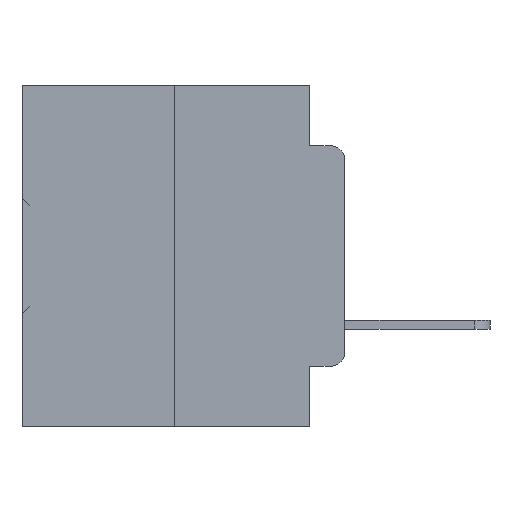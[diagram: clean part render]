
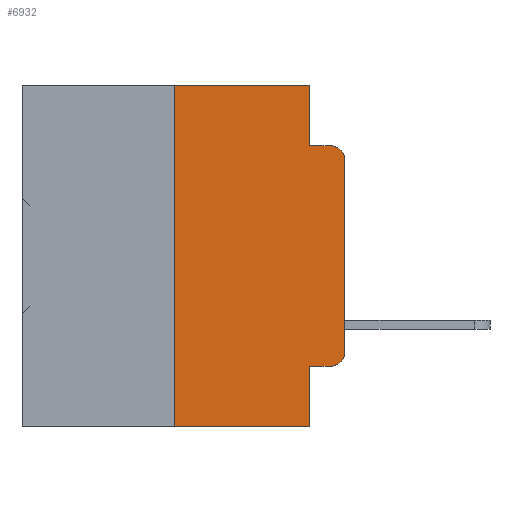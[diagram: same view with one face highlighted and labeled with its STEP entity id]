
A CAD part, left-side view. The second image highlights one B-rep face of the part: STEP entity #6932.
In plain terms, the highlighted planar face has unit normal (-1, 0, 0).
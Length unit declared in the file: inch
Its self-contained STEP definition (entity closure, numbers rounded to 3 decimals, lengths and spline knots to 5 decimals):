
#1112 = ORIENTED_EDGE ( 'NONE', *, *, #26178, .T. ) ;
#2345 = CARTESIAN_POINT ( 'NONE',  ( 0., 0.051, -0.0885 ) ) ;
#2995 = EDGE_CURVE ( 'NONE', #19259, #22812, #21436, .T. ) ;
#3090 = DIRECTION ( 'NONE',  ( 0., 0., -1. ) ) ;
#3223 = ORIENTED_EDGE ( 'NONE', *, *, #34091, .F. ) ;
#3298 = VECTOR ( 'NONE', #9913, 39.37008 ) ;
#3978 = CARTESIAN_POINT ( 'NONE',  ( 0., 0.051, 0. ) ) ;
#4109 = VECTOR ( 'NONE', #13812, 39.37008 ) ;
#4898 = CARTESIAN_POINT ( 'NONE',  ( 0., 0.25, 0. ) ) ;
#5034 = EDGE_CURVE ( 'NONE', #5572, #13903, #10807, .T. ) ;
#5572 = VERTEX_POINT ( 'NONE', #36904 ) ;
#5828 = CARTESIAN_POINT ( 'NONE',  ( 0., 0.25, -0.5 ) ) ;
#6393 = CARTESIAN_POINT ( 'NONE',  ( 0., 0.051, -0.4115 ) ) ;
#6932 = ADVANCED_FACE ( 'NONE', ( #32991 ), #20229, .F. ) ;
#7000 = DIRECTION ( 'NONE',  ( 0., 0., -1. ) ) ;
#7051 = EDGE_CURVE ( 'NONE', #13903, #15037, #23560, .T. ) ;
#7259 = CARTESIAN_POINT ( 'NONE',  ( 0., 0.051, -0.5 ) ) ;
#7495 = AXIS2_PLACEMENT_3D ( 'NONE', #26180, #7966, #29075 ) ;
#7966 = DIRECTION ( 'NONE',  ( 1., 0., 0. ) ) ;
#8162 = CARTESIAN_POINT ( 'NONE',  ( 0., 0.051, -0.4115 ) ) ;
#8817 = ORIENTED_EDGE ( 'NONE', *, *, #2995, .F. ) ;
#9519 = DIRECTION ( 'NONE',  ( 0., -1., 0. ) ) ;
#9913 = DIRECTION ( 'NONE',  ( 0., -1., 0. ) ) ;
#9925 = CARTESIAN_POINT ( 'NONE',  ( 0., 0., -0.3915 ) ) ;
#10504 = DIRECTION ( 'NONE',  ( 0., 0., -1. ) ) ;
#10753 = CARTESIAN_POINT ( 'NONE',  ( 0., 0.473, 0. ) ) ;
#10807 = LINE ( 'NONE', #3978, #38237 ) ;
#11054 = ORIENTED_EDGE ( 'NONE', *, *, #7051, .F. ) ;
#11085 = CARTESIAN_POINT ( 'NONE',  ( 0., 0.02, -0.0885 ) ) ;
#11275 = EDGE_CURVE ( 'NONE', #12310, #15037, #15644, .T. ) ;
#11623 = ORIENTED_EDGE ( 'NONE', *, *, #32416, .T. ) ;
#12310 = VERTEX_POINT ( 'NONE', #19787 ) ;
#12954 = ORIENTED_EDGE ( 'NONE', *, *, #35680, .F. ) ;
#13291 = EDGE_CURVE ( 'NONE', #30550, #12310, #13988, .T. ) ;
#13812 = DIRECTION ( 'NONE',  ( 0., -1., 0. ) ) ;
#13903 = VERTEX_POINT ( 'NONE', #28449 ) ;
#13988 = LINE ( 'NONE', #23519, #20225 ) ;
#14343 = CARTESIAN_POINT ( 'NONE',  ( 0., 0.02, -0.1085 ) ) ;
#14706 = LINE ( 'NONE', #6393, #29610 ) ;
#14971 = DIRECTION ( 'NONE',  ( 0., 0., 1. ) ) ;
#15037 = VERTEX_POINT ( 'NONE', #11085 ) ;
#15644 = CIRCLE ( 'NONE', #25232, 0.02 ) ;
#15967 = CARTESIAN_POINT ( 'NONE',  ( 0., 0.473, -0.5 ) ) ;
#17456 = DIRECTION ( 'NONE',  ( 0., 0., -1. ) ) ;
#17955 = ORIENTED_EDGE ( 'NONE', *, *, #5034, .F. ) ;
#19259 = VERTEX_POINT ( 'NONE', #5828 ) ;
#19607 = CARTESIAN_POINT ( 'NONE',  ( 0., 0.051, 0. ) ) ;
#19787 = CARTESIAN_POINT ( 'NONE',  ( 0., 0., -0.1085 ) ) ;
#20137 = EDGE_LOOP ( 'NONE', ( #28107, #32117, #11054, #17955, #3223, #8817, #11623, #12954, #25968, #1112 ) ) ;
#20225 = VECTOR ( 'NONE', #32173, 39.37008 ) ;
#20229 = PLANE ( 'NONE',  #7495 ) ;
#21436 = LINE ( 'NONE', #29788, #35810 ) ;
#21439 = DIRECTION ( 'NONE',  ( -1., 0., 0. ) ) ;
#21669 = VECTOR ( 'NONE', #26565, 39.37008 ) ;
#21967 = CARTESIAN_POINT ( 'NONE',  ( 0., 0.02, -0.4115 ) ) ;
#22170 = VECTOR ( 'NONE', #10504, 39.37008 ) ;
#22812 = VERTEX_POINT ( 'NONE', #4898 ) ;
#23519 = CARTESIAN_POINT ( 'NONE',  ( 0., 0., 0. ) ) ;
#23560 = LINE ( 'NONE', #2345, #21669 ) ;
#25232 = AXIS2_PLACEMENT_3D ( 'NONE', #14343, #34882, #17456 ) ;
#25968 = ORIENTED_EDGE ( 'NONE', *, *, #33820, .T. ) ;
#25975 = VERTEX_POINT ( 'NONE', #8162 ) ;
#26178 = EDGE_CURVE ( 'NONE', #35532, #30550, #36052, .T. ) ;
#26180 = CARTESIAN_POINT ( 'NONE',  ( 0., 0.473, 0. ) ) ;
#26565 = DIRECTION ( 'NONE',  ( 0., -1., 0. ) ) ;
#28107 = ORIENTED_EDGE ( 'NONE', *, *, #13291, .T. ) ;
#28263 = LINE ( 'NONE', #10753, #4109 ) ;
#28449 = CARTESIAN_POINT ( 'NONE',  ( 0., 0.051, -0.0885 ) ) ;
#29075 = DIRECTION ( 'NONE',  ( 0., 0., -1. ) ) ;
#29610 = VECTOR ( 'NONE', #9519, 39.37008 ) ;
#29788 = CARTESIAN_POINT ( 'NONE',  ( 0., 0.25, 0. ) ) ;
#29891 = LINE ( 'NONE', #19607, #22170 ) ;
#30550 = VERTEX_POINT ( 'NONE', #9925 ) ;
#32117 = ORIENTED_EDGE ( 'NONE', *, *, #11275, .T. ) ;
#32173 = DIRECTION ( 'NONE',  ( 0., 0., 1. ) ) ;
#32416 = EDGE_CURVE ( 'NONE', #19259, #37397, #35884, .T. ) ;
#32991 = FACE_OUTER_BOUND ( 'NONE', #20137, .T. ) ;
#33820 = EDGE_CURVE ( 'NONE', #25975, #35532, #14706, .T. ) ;
#34091 = EDGE_CURVE ( 'NONE', #22812, #5572, #28263, .T. ) ;
#34882 = DIRECTION ( 'NONE',  ( -1., 0., 0. ) ) ;
#35532 = VERTEX_POINT ( 'NONE', #21967 ) ;
#35680 = EDGE_CURVE ( 'NONE', #25975, #37397, #29891, .T. ) ;
#35810 = VECTOR ( 'NONE', #14971, 39.37008 ) ;
#35884 = LINE ( 'NONE', #15967, #3298 ) ;
#36052 = CIRCLE ( 'NONE', #37141, 0.02 ) ;
#36904 = CARTESIAN_POINT ( 'NONE',  ( 0., 0.051, 0. ) ) ;
#37141 = AXIS2_PLACEMENT_3D ( 'NONE', #38485, #21439, #3090 ) ;
#37397 = VERTEX_POINT ( 'NONE', #7259 ) ;
#38237 = VECTOR ( 'NONE', #7000, 39.37008 ) ;
#38485 = CARTESIAN_POINT ( 'NONE',  ( 0., 0.02, -0.3915 ) ) ;
